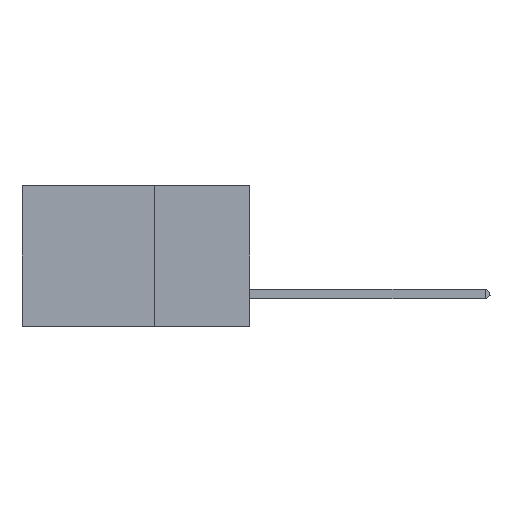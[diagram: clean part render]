
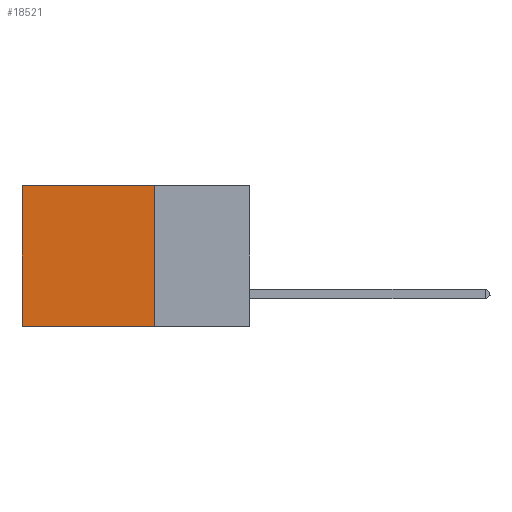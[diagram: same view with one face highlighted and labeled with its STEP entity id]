
A CAD part, left-side view. The second image highlights one B-rep face of the part: STEP entity #18521.
In plain terms, the highlighted planar face has unit normal (-1, 0, 0).
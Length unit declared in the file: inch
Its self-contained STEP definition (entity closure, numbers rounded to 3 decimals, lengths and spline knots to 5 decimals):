
#754 = CARTESIAN_POINT ( 'NONE',  ( 0.2875, 0.25, -0.37 ) ) ;
#3215 = CARTESIAN_POINT ( 'NONE',  ( 0.2875, 0.6, 0. ) ) ;
#3439 = LINE ( 'NONE', #35756, #37505 ) ;
#4757 = VERTEX_POINT ( 'NONE', #10744 ) ;
#5153 = VECTOR ( 'NONE', #7398, 39.37008 ) ;
#6257 = EDGE_LOOP ( 'NONE', ( #16088, #29380, #19635, #34693 ) ) ;
#7398 = DIRECTION ( 'NONE',  ( 0., 1., 0. ) ) ;
#8888 = EDGE_CURVE ( 'NONE', #21265, #4757, #24181, .T. ) ;
#10356 = VECTOR ( 'NONE', #16361, 39.37008 ) ;
#10744 = CARTESIAN_POINT ( 'NONE',  ( 0.2875, 0.6, -0.37 ) ) ;
#12271 = AXIS2_PLACEMENT_3D ( 'NONE', #19518, #32515, #22689 ) ;
#13728 = EDGE_CURVE ( 'NONE', #31228, #33506, #25132, .T. ) ;
#16088 = ORIENTED_EDGE ( 'NONE', *, *, #20330, .T. ) ;
#16361 = DIRECTION ( 'NONE',  ( 0., 0., -1. ) ) ;
#16590 = CARTESIAN_POINT ( 'NONE',  ( 0.2875, 0.25, 0. ) ) ;
#16995 = CARTESIAN_POINT ( 'NONE',  ( 0.2875, 0.25, 0. ) ) ;
#17403 = VECTOR ( 'NONE', #36633, 39.37008 ) ;
#18521 = ADVANCED_FACE ( 'NONE', ( #19825 ), #42189, .F. ) ;
#19518 = CARTESIAN_POINT ( 'NONE',  ( 0.2875, 0.25, 0. ) ) ;
#19635 = ORIENTED_EDGE ( 'NONE', *, *, #39203, .F. ) ;
#19825 = FACE_OUTER_BOUND ( 'NONE', #6257, .T. ) ;
#20330 = EDGE_CURVE ( 'NONE', #33506, #4757, #23716, .T. ) ;
#21265 = VERTEX_POINT ( 'NONE', #41527 ) ;
#22689 = DIRECTION ( 'NONE',  ( 0., 0., -1. ) ) ;
#23019 = DIRECTION ( 'NONE',  ( 0., 0., -1. ) ) ;
#23716 = LINE ( 'NONE', #3215, #10356 ) ;
#24181 = LINE ( 'NONE', #754, #5153 ) ;
#25132 = LINE ( 'NONE', #16995, #17403 ) ;
#29380 = ORIENTED_EDGE ( 'NONE', *, *, #8888, .F. ) ;
#31228 = VERTEX_POINT ( 'NONE', #16590 ) ;
#32515 = DIRECTION ( 'NONE',  ( 1., 0., 0. ) ) ;
#33506 = VERTEX_POINT ( 'NONE', #39058 ) ;
#34693 = ORIENTED_EDGE ( 'NONE', *, *, #13728, .T. ) ;
#35756 = CARTESIAN_POINT ( 'NONE',  ( 0.2875, 0.25, 0. ) ) ;
#36633 = DIRECTION ( 'NONE',  ( 0., 1., 0. ) ) ;
#37505 = VECTOR ( 'NONE', #23019, 39.37008 ) ;
#39058 = CARTESIAN_POINT ( 'NONE',  ( 0.2875, 0.6, 0. ) ) ;
#39203 = EDGE_CURVE ( 'NONE', #31228, #21265, #3439, .T. ) ;
#41527 = CARTESIAN_POINT ( 'NONE',  ( 0.2875, 0.25, -0.37 ) ) ;
#42189 = PLANE ( 'NONE',  #12271 ) ;
